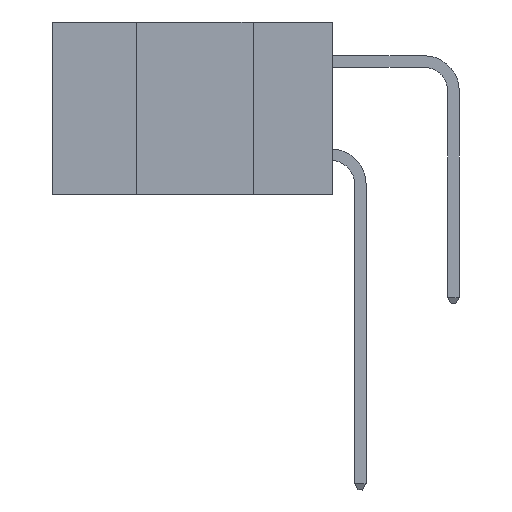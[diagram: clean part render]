
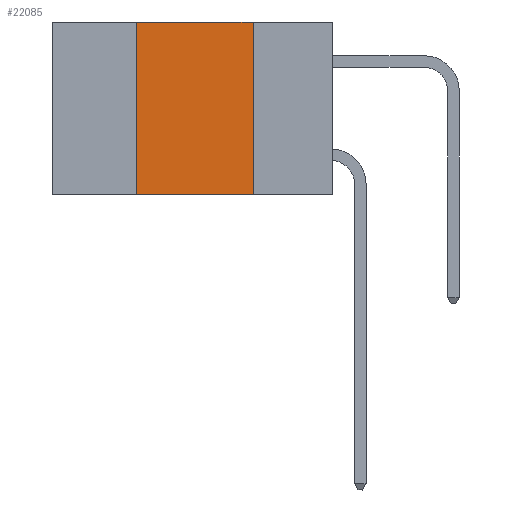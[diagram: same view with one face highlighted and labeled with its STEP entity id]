
A CAD part, left-side view. The second image highlights one B-rep face of the part: STEP entity #22085.
In plain terms, the highlighted planar face has unit normal (-1, 0, 0).
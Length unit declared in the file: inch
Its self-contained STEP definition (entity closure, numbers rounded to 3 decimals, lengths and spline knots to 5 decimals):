
#1012 = CARTESIAN_POINT ( 'NONE',  ( 0., 0.42, 0. ) ) ;
#1217 = ORIENTED_EDGE ( 'NONE', *, *, #24620, .F. ) ;
#1512 = VERTEX_POINT ( 'NONE', #27370 ) ;
#2259 = PLANE ( 'NONE',  #16264 ) ;
#2361 = LINE ( 'NONE', #8555, #12774 ) ;
#2608 = LINE ( 'NONE', #6875, #8997 ) ;
#2687 = DIRECTION ( 'NONE',  ( 1., 0., 0. ) ) ;
#2718 = EDGE_CURVE ( 'NONE', #18043, #9161, #2608, .T. ) ;
#2825 = FACE_OUTER_BOUND ( 'NONE', #10568, .T. ) ;
#3649 = VECTOR ( 'NONE', #3942, 39.37008 ) ;
#3942 = DIRECTION ( 'NONE',  ( 0., -1., 0. ) ) ;
#5585 = CARTESIAN_POINT ( 'NONE',  ( 0., 0.42, -0.37 ) ) ;
#6139 = CARTESIAN_POINT ( 'NONE',  ( 0., 0.6, 0. ) ) ;
#6875 = CARTESIAN_POINT ( 'NONE',  ( 0., 0.6, -0.37 ) ) ;
#7148 = DIRECTION ( 'NONE',  ( 0., -1., 0. ) ) ;
#7471 = EDGE_CURVE ( 'NONE', #18043, #15595, #19655, .T. ) ;
#8555 = CARTESIAN_POINT ( 'NONE',  ( 0., 0.17, -0.37 ) ) ;
#8997 = VECTOR ( 'NONE', #7148, 39.37008 ) ;
#9161 = VERTEX_POINT ( 'NONE', #22235 ) ;
#10568 = EDGE_LOOP ( 'NONE', ( #29049, #1217, #14271, #17083 ) ) ;
#12774 = VECTOR ( 'NONE', #15478, 39.37008 ) ;
#13581 = CARTESIAN_POINT ( 'NONE',  ( 0., 0.6, 0. ) ) ;
#14271 = ORIENTED_EDGE ( 'NONE', *, *, #7471, .F. ) ;
#15303 = EDGE_CURVE ( 'NONE', #1512, #9161, #2361, .T. ) ;
#15478 = DIRECTION ( 'NONE',  ( 0., 0., -1. ) ) ;
#15595 = VERTEX_POINT ( 'NONE', #1012 ) ;
#16264 = AXIS2_PLACEMENT_3D ( 'NONE', #13581, #2687, #20222 ) ;
#17083 = ORIENTED_EDGE ( 'NONE', *, *, #2718, .T. ) ;
#17344 = LINE ( 'NONE', #6139, #3649 ) ;
#18043 = VERTEX_POINT ( 'NONE', #5585 ) ;
#19655 = LINE ( 'NONE', #28671, #20996 ) ;
#20222 = DIRECTION ( 'NONE',  ( 0., 0., -1. ) ) ;
#20996 = VECTOR ( 'NONE', #24778, 39.37008 ) ;
#22085 = ADVANCED_FACE ( 'NONE', ( #2825 ), #2259, .F. ) ;
#22235 = CARTESIAN_POINT ( 'NONE',  ( 0., 0.17, -0.37 ) ) ;
#24620 = EDGE_CURVE ( 'NONE', #15595, #1512, #17344, .T. ) ;
#24778 = DIRECTION ( 'NONE',  ( 0., 0., 1. ) ) ;
#27370 = CARTESIAN_POINT ( 'NONE',  ( 0., 0.17, 0. ) ) ;
#28671 = CARTESIAN_POINT ( 'NONE',  ( 0., 0.42, -0.37 ) ) ;
#29049 = ORIENTED_EDGE ( 'NONE', *, *, #15303, .F. ) ;
